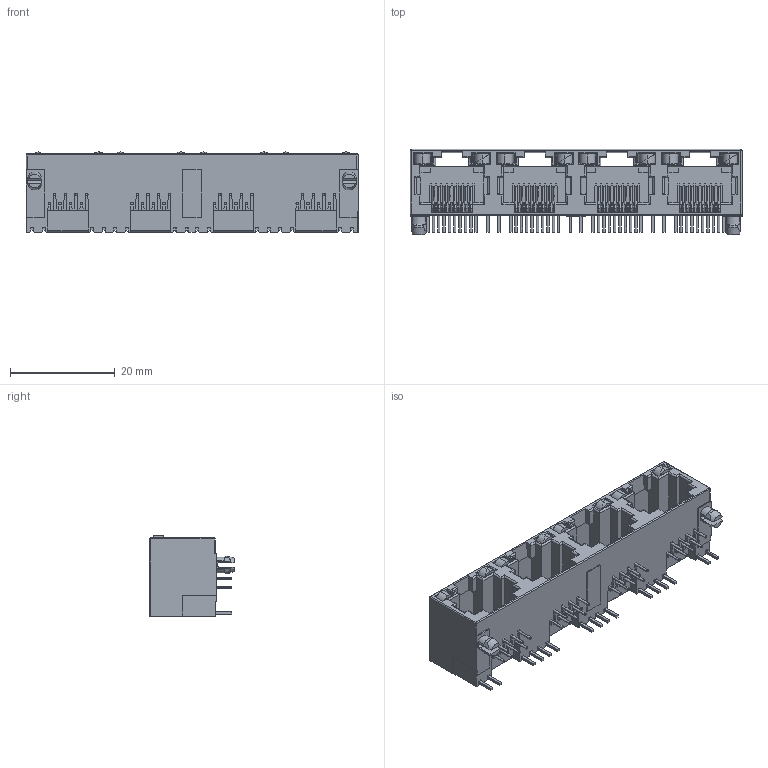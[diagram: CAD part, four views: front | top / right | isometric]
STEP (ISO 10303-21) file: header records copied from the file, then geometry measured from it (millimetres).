
FILE_DESCRIPTION (( 'STEP AP203' ), '1' );
FILE_NAME ('J67048822N15011.STEP', '2020-03-20T13:07:23', ( '' ), ( '' ), 'SwSTEP 2.0', 'SolidWorks 2016', '' );
FILE_SCHEMA (( 'CONFIG_CONTROL_DESIGN' ));
Length unit declared in the file: millimetre
Products named in the file (5): J67048822N15011; 67 Contacts; 67 Insulator; 67 LED RH_5-Green-Yellow; 67 LED LH_1-Yellow
Assembly tree (13 placements, depth 2):
  J67048822N15011
    67 Insulator
    67 Contacts  x4
    67 LED LH_1-Yellow  x4
    67 LED RH_5-Green-Yellow  x4
Bounding box: 63.3 x 16.25 x 15.28 mm (x, y, z)
Volume: 5159.3 mm3; surface area: 11572.8 mm2
Topology: 41 solids, 41 shells, 2473 faces, 6556 edges, 4100 vertices
Faces by surface type: plane 1781, cylinder 484, bspline 200, cone 8
Entity records: 62432 total; most frequent: CARTESIAN_POINT 12233, ORIENTED_EDGE 10786, DIRECTION 9581, EDGE_CURVE 5393, LINE 4683, VECTOR 4683, VERTEX_POINT 3365, AXIS2_PLACEMENT_3D 2449
